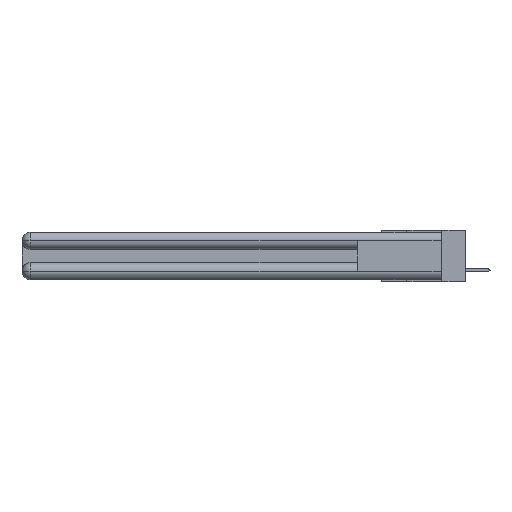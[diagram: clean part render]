
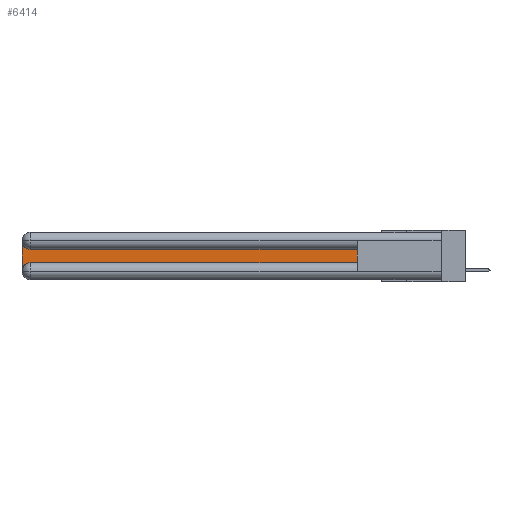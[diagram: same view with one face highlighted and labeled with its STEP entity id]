
A CAD part, left-side view. The second image highlights one B-rep face of the part: STEP entity #6414.
In plain terms, the highlighted planar face has unit normal (-1, 0, 0).
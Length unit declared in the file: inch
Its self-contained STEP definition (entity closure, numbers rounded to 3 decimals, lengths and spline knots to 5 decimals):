
#1872 = VERTEX_POINT ( 'NONE', #18922 ) ;
#2337 = ORIENTED_EDGE ( 'NONE', *, *, #17649, .T. ) ;
#3802 = DIRECTION ( 'NONE',  ( 1., 0., 0. ) ) ;
#4347 = CARTESIAN_POINT ( 'NONE',  ( 0.075, 0.6, -0.2175 ) ) ;
#5540 = LINE ( 'NONE', #23235, #15459 ) ;
#6361 = DIRECTION ( 'NONE',  ( 1., 0., 0. ) ) ;
#6414 = ADVANCED_FACE ( 'NONE', ( #12473 ), #16590, .F. ) ;
#8153 = CARTESIAN_POINT ( 'NONE',  ( 0.075, 3., -0.0625 ) ) ;
#8184 = DIRECTION ( 'NONE',  ( 0., 0., -1. ) ) ;
#8550 = ORIENTED_EDGE ( 'NONE', *, *, #10822, .T. ) ;
#9962 = AXIS2_PLACEMENT_3D ( 'NONE', #23052, #14309, #8184 ) ;
#10310 = CARTESIAN_POINT ( 'NONE',  ( 0.075, 2.94, -0.2775 ) ) ;
#10822 = EDGE_CURVE ( 'NONE', #13514, #16993, #5540, .T. ) ;
#11182 = EDGE_CURVE ( 'NONE', #17507, #20492, #26468, .T. ) ;
#11386 = DIRECTION ( 'NONE',  ( 0., 0., -1. ) ) ;
#11800 = EDGE_CURVE ( 'NONE', #19381, #17507, #13869, .T. ) ;
#12102 = ORIENTED_EDGE ( 'NONE', *, *, #11800, .T. ) ;
#12473 = FACE_OUTER_BOUND ( 'NONE', #20034, .T. ) ;
#12741 = DIRECTION ( 'NONE',  ( 0., 0., -1. ) ) ;
#13303 = ORIENTED_EDGE ( 'NONE', *, *, #20967, .T. ) ;
#13514 = VERTEX_POINT ( 'NONE', #20020 ) ;
#13869 = CIRCLE ( 'NONE', #17137, 0.06 ) ;
#14309 = DIRECTION ( 'NONE',  ( 1., 0., 0. ) ) ;
#14628 = DIRECTION ( 'NONE',  ( 0., 1., 0. ) ) ;
#15016 = DIRECTION ( 'NONE',  ( 0., 0., 1. ) ) ;
#15224 = VECTOR ( 'NONE', #11386, 39.37008 ) ;
#15459 = VECTOR ( 'NONE', #21208, 39.37008 ) ;
#16590 = PLANE ( 'NONE',  #9962 ) ;
#16993 = VERTEX_POINT ( 'NONE', #18030 ) ;
#17137 = AXIS2_PLACEMENT_3D ( 'NONE', #25412, #6361, #12741 ) ;
#17507 = VERTEX_POINT ( 'NONE', #8153 ) ;
#17649 = EDGE_CURVE ( 'NONE', #20492, #13514, #23793, .T. ) ;
#17936 = CARTESIAN_POINT ( 'NONE',  ( 0.075, 3., -0.2175 ) ) ;
#18030 = CARTESIAN_POINT ( 'NONE',  ( 0.075, 0.6, -0.2175 ) ) ;
#18355 = LINE ( 'NONE', #20803, #20669 ) ;
#18922 = CARTESIAN_POINT ( 'NONE',  ( 0.075, 0.6, -0.1225 ) ) ;
#18995 = LINE ( 'NONE', #4347, #20627 ) ;
#19381 = VERTEX_POINT ( 'NONE', #19476 ) ;
#19476 = CARTESIAN_POINT ( 'NONE',  ( 0.075, 2.94, -0.1225 ) ) ;
#20020 = CARTESIAN_POINT ( 'NONE',  ( 0.075, 2.94, -0.2175 ) ) ;
#20034 = EDGE_LOOP ( 'NONE', ( #13303, #12102, #23710, #2337, #8550, #25454 ) ) ;
#20492 = VERTEX_POINT ( 'NONE', #22470 ) ;
#20627 = VECTOR ( 'NONE', #15016, 39.37008 ) ;
#20669 = VECTOR ( 'NONE', #14628, 39.37008 ) ;
#20803 = CARTESIAN_POINT ( 'NONE',  ( 0.075, 0.6, -0.1225 ) ) ;
#20967 = EDGE_CURVE ( 'NONE', #1872, #19381, #18355, .T. ) ;
#21208 = DIRECTION ( 'NONE',  ( 0., -1., 0. ) ) ;
#22470 = CARTESIAN_POINT ( 'NONE',  ( 0.075, 3., -0.2775 ) ) ;
#23052 = CARTESIAN_POINT ( 'NONE',  ( 0.075, 3., -0.1225 ) ) ;
#23235 = CARTESIAN_POINT ( 'NONE',  ( 0.075, 0.6, -0.2175 ) ) ;
#23710 = ORIENTED_EDGE ( 'NONE', *, *, #11182, .T. ) ;
#23793 = CIRCLE ( 'NONE', #25188, 0.06 ) ;
#25098 = DIRECTION ( 'NONE',  ( 0., 0., -1. ) ) ;
#25188 = AXIS2_PLACEMENT_3D ( 'NONE', #10310, #3802, #25098 ) ;
#25412 = CARTESIAN_POINT ( 'NONE',  ( 0.075, 2.94, -0.0625 ) ) ;
#25454 = ORIENTED_EDGE ( 'NONE', *, *, #26576, .T. ) ;
#26468 = LINE ( 'NONE', #17936, #15224 ) ;
#26576 = EDGE_CURVE ( 'NONE', #16993, #1872, #18995, .T. ) ;
